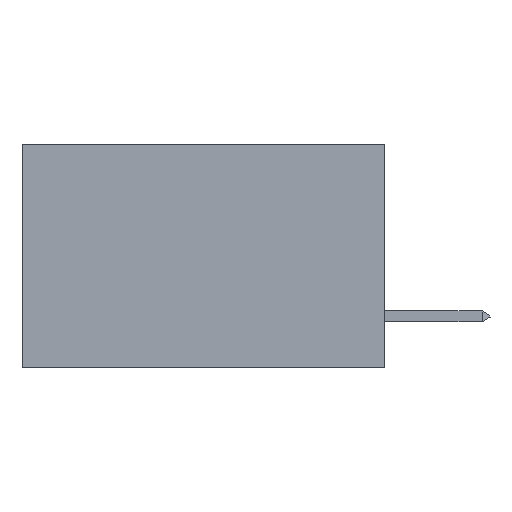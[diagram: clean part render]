
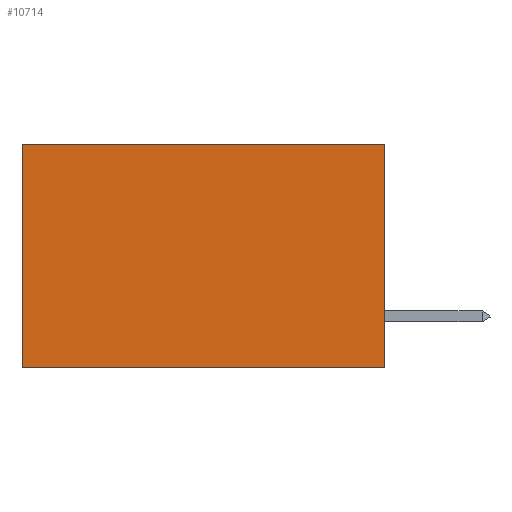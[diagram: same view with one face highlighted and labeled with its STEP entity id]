
A CAD part, left-side view. The second image highlights one B-rep face of the part: STEP entity #10714.
In plain terms, the highlighted planar face has unit normal (-1, 0, 0).
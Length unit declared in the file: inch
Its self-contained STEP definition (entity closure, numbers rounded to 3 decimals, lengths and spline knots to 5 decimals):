
#402 = CARTESIAN_POINT ( 'NONE',  ( 0.2875, 0., 0. ) ) ;
#1220 = VERTEX_POINT ( 'NONE', #21971 ) ;
#2730 = CARTESIAN_POINT ( 'NONE',  ( 0.2875, 0., 0. ) ) ;
#2878 = PLANE ( 'NONE',  #37056 ) ;
#3480 = VERTEX_POINT ( 'NONE', #30328 ) ;
#3830 = DIRECTION ( 'NONE',  ( 0., 1., 0. ) ) ;
#5929 = CARTESIAN_POINT ( 'NONE',  ( 0.2875, 0.6, 0. ) ) ;
#7522 = EDGE_CURVE ( 'NONE', #37751, #1220, #34009, .T. ) ;
#7877 = DIRECTION ( 'NONE',  ( 0., 0., -1. ) ) ;
#8548 = ORIENTED_EDGE ( 'NONE', *, *, #32921, .F. ) ;
#10714 = ADVANCED_FACE ( 'NONE', ( #35195 ), #2878, .F. ) ;
#12724 = DIRECTION ( 'NONE',  ( 1., 0., 0. ) ) ;
#13167 = EDGE_CURVE ( 'NONE', #37751, #26390, #28260, .T. ) ;
#13353 = ORIENTED_EDGE ( 'NONE', *, *, #7522, .F. ) ;
#15826 = CARTESIAN_POINT ( 'NONE',  ( 0.2875, 0., 0. ) ) ;
#16034 = VECTOR ( 'NONE', #3830, 39.37008 ) ;
#16845 = EDGE_CURVE ( 'NONE', #26390, #3480, #24773, .T. ) ;
#21260 = CARTESIAN_POINT ( 'NONE',  ( 0.2875, 0.6, 0. ) ) ;
#21971 = CARTESIAN_POINT ( 'NONE',  ( 0.2875, 0., -0.37 ) ) ;
#24312 = DIRECTION ( 'NONE',  ( 0., 1., 0. ) ) ;
#24773 = LINE ( 'NONE', #5929, #40518 ) ;
#25442 = EDGE_LOOP ( 'NONE', ( #43454, #8548, #13353, #34323 ) ) ;
#25956 = LINE ( 'NONE', #40925, #41156 ) ;
#26390 = VERTEX_POINT ( 'NONE', #21260 ) ;
#28183 = CARTESIAN_POINT ( 'NONE',  ( 0.2875, 0., 0. ) ) ;
#28260 = LINE ( 'NONE', #402, #16034 ) ;
#30328 = CARTESIAN_POINT ( 'NONE',  ( 0.2875, 0.6, -0.37 ) ) ;
#32921 = EDGE_CURVE ( 'NONE', #1220, #3480, #25956, .T. ) ;
#34009 = LINE ( 'NONE', #28183, #40811 ) ;
#34323 = ORIENTED_EDGE ( 'NONE', *, *, #13167, .T. ) ;
#35195 = FACE_OUTER_BOUND ( 'NONE', #25442, .T. ) ;
#36663 = DIRECTION ( 'NONE',  ( 0., 0., -1. ) ) ;
#37056 = AXIS2_PLACEMENT_3D ( 'NONE', #2730, #12724, #43382 ) ;
#37751 = VERTEX_POINT ( 'NONE', #15826 ) ;
#40518 = VECTOR ( 'NONE', #36663, 39.37008 ) ;
#40811 = VECTOR ( 'NONE', #7877, 39.37008 ) ;
#40925 = CARTESIAN_POINT ( 'NONE',  ( 0.2875, 0., -0.37 ) ) ;
#41156 = VECTOR ( 'NONE', #24312, 39.37008 ) ;
#43382 = DIRECTION ( 'NONE',  ( 0., 0., -1. ) ) ;
#43454 = ORIENTED_EDGE ( 'NONE', *, *, #16845, .T. ) ;
